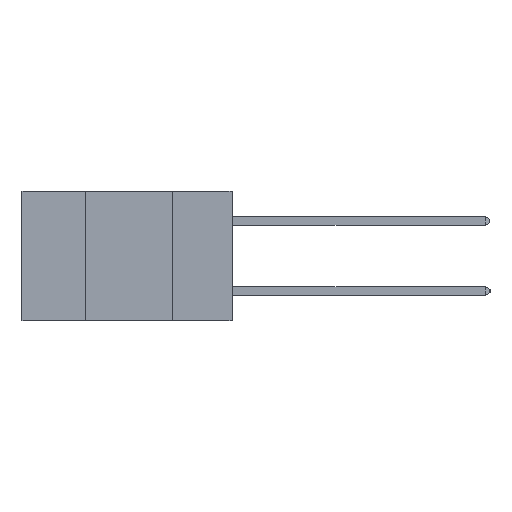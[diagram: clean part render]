
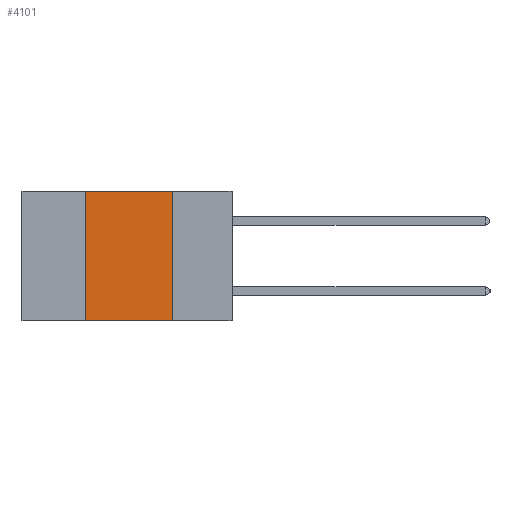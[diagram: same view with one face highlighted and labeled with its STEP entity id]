
A CAD part, left-side view. The second image highlights one B-rep face of the part: STEP entity #4101.
In plain terms, the highlighted planar face has unit normal (-1, 0, 0).
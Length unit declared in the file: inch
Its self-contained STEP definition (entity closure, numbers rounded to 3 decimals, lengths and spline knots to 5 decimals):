
#9 = EDGE_CURVE ( 'NONE', #13597, #3810, #17775, .T. ) ;
#435 = LINE ( 'NONE', #17869, #7898 ) ;
#1047 = EDGE_CURVE ( 'NONE', #13597, #3349, #4921, .T. ) ;
#1745 = EDGE_LOOP ( 'NONE', ( #10243, #16548, #10702, #7438 ) ) ;
#2416 = EDGE_CURVE ( 'NONE', #3810, #8375, #435, .T. ) ;
#3349 = VERTEX_POINT ( 'NONE', #5590 ) ;
#3810 = VERTEX_POINT ( 'NONE', #13347 ) ;
#4101 = ADVANCED_FACE ( 'NONE', ( #15543 ), #9099, .F. ) ;
#4773 = CARTESIAN_POINT ( 'NONE',  ( 0., 0.42, 0. ) ) ;
#4921 = LINE ( 'NONE', #15442, #8438 ) ;
#5021 = DIRECTION ( 'NONE',  ( 0., -1., 0. ) ) ;
#5590 = CARTESIAN_POINT ( 'NONE',  ( 0., 0.17, -0.37 ) ) ;
#5898 = VECTOR ( 'NONE', #9078, 39.37008 ) ;
#5996 = LINE ( 'NONE', #6266, #13929 ) ;
#6075 = DIRECTION ( 'NONE',  ( 0., 0., -1. ) ) ;
#6266 = CARTESIAN_POINT ( 'NONE',  ( 0., 0.17, 0. ) ) ;
#6915 = CARTESIAN_POINT ( 'NONE',  ( 0., 0.6, 0. ) ) ;
#7438 = ORIENTED_EDGE ( 'NONE', *, *, #1047, .T. ) ;
#7898 = VECTOR ( 'NONE', #18204, 39.37008 ) ;
#8130 = AXIS2_PLACEMENT_3D ( 'NONE', #6915, #9901, #6075 ) ;
#8375 = VERTEX_POINT ( 'NONE', #11912 ) ;
#8438 = VECTOR ( 'NONE', #5021, 39.37008 ) ;
#9025 = EDGE_CURVE ( 'NONE', #8375, #3349, #5996, .T. ) ;
#9078 = DIRECTION ( 'NONE',  ( 0., 0., 1. ) ) ;
#9099 = PLANE ( 'NONE',  #8130 ) ;
#9901 = DIRECTION ( 'NONE',  ( 1., 0., 0. ) ) ;
#10243 = ORIENTED_EDGE ( 'NONE', *, *, #9025, .F. ) ;
#10702 = ORIENTED_EDGE ( 'NONE', *, *, #9, .F. ) ;
#11912 = CARTESIAN_POINT ( 'NONE',  ( 0., 0.17, 0. ) ) ;
#13347 = CARTESIAN_POINT ( 'NONE',  ( 0., 0.42, 0. ) ) ;
#13597 = VERTEX_POINT ( 'NONE', #17322 ) ;
#13929 = VECTOR ( 'NONE', #16641, 39.37008 ) ;
#15442 = CARTESIAN_POINT ( 'NONE',  ( 0., 0.6, -0.37 ) ) ;
#15543 = FACE_OUTER_BOUND ( 'NONE', #1745, .T. ) ;
#16548 = ORIENTED_EDGE ( 'NONE', *, *, #2416, .F. ) ;
#16641 = DIRECTION ( 'NONE',  ( 0., 0., -1. ) ) ;
#17322 = CARTESIAN_POINT ( 'NONE',  ( 0., 0.42, -0.37 ) ) ;
#17775 = LINE ( 'NONE', #4773, #5898 ) ;
#17869 = CARTESIAN_POINT ( 'NONE',  ( 0., 0.6, 0. ) ) ;
#18204 = DIRECTION ( 'NONE',  ( 0., -1., 0. ) ) ;
